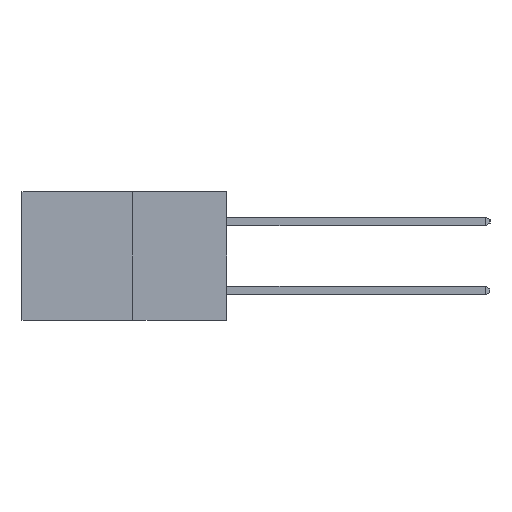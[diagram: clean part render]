
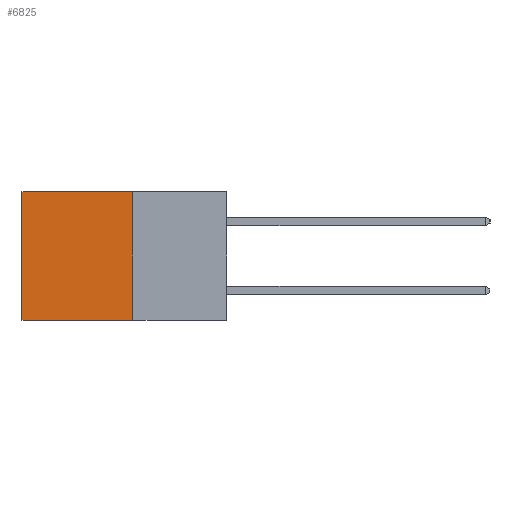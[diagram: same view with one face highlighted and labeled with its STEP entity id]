
A CAD part, left-side view. The second image highlights one B-rep face of the part: STEP entity #6825.
In plain terms, the highlighted planar face has unit normal (-1, 0, 0).
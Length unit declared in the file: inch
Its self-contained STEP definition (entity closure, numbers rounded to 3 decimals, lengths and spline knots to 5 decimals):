
#416 = DIRECTION ( 'NONE',  ( 0., 0., -1. ) ) ;
#569 = VECTOR ( 'NONE', #416, 39.37008 ) ;
#786 = ORIENTED_EDGE ( 'NONE', *, *, #5206, .T. ) ;
#916 = CARTESIAN_POINT ( 'NONE',  ( 0.277, 0.59, 0. ) ) ;
#1398 = VERTEX_POINT ( 'NONE', #5485 ) ;
#1598 = VECTOR ( 'NONE', #9127, 39.37008 ) ;
#1998 = LINE ( 'NONE', #2437, #10944 ) ;
#2204 = DIRECTION ( 'NONE',  ( 0., 1., 0. ) ) ;
#2437 = CARTESIAN_POINT ( 'NONE',  ( 0.277, 0.27, 0. ) ) ;
#2507 = DIRECTION ( 'NONE',  ( 0., 0., -1. ) ) ;
#2519 = DIRECTION ( 'NONE',  ( 1., 0., 0. ) ) ;
#2529 = PLANE ( 'NONE',  #3953 ) ;
#2538 = CARTESIAN_POINT ( 'NONE',  ( 0.277, 0.27, -0.37 ) ) ;
#2888 = ORIENTED_EDGE ( 'NONE', *, *, #8883, .T. ) ;
#3163 = CARTESIAN_POINT ( 'NONE',  ( 0.277, 0.59, -0.37 ) ) ;
#3779 = CARTESIAN_POINT ( 'NONE',  ( 0.277, 0.27, -0.37 ) ) ;
#3953 = AXIS2_PLACEMENT_3D ( 'NONE', #2538, #2519, #2507 ) ;
#4149 = ORIENTED_EDGE ( 'NONE', *, *, #7336, .F. ) ;
#4324 = LINE ( 'NONE', #5685, #1598 ) ;
#5206 = EDGE_CURVE ( 'NONE', #1398, #8632, #1998, .T. ) ;
#5485 = CARTESIAN_POINT ( 'NONE',  ( 0.277, 0.27, 0. ) ) ;
#5685 = CARTESIAN_POINT ( 'NONE',  ( 0.277, 0.59, -0.37 ) ) ;
#6700 = VERTEX_POINT ( 'NONE', #3163 ) ;
#6825 = ADVANCED_FACE ( 'NONE', ( #10793 ), #2529, .F. ) ;
#7336 = EDGE_CURVE ( 'NONE', #1398, #9811, #7734, .T. ) ;
#7734 = LINE ( 'NONE', #10943, #569 ) ;
#7762 = CARTESIAN_POINT ( 'NONE',  ( 0.277, 0.27, -0.37 ) ) ;
#8063 = ORIENTED_EDGE ( 'NONE', *, *, #10306, .F. ) ;
#8097 = LINE ( 'NONE', #7762, #10122 ) ;
#8632 = VERTEX_POINT ( 'NONE', #916 ) ;
#8643 = DIRECTION ( 'NONE',  ( 0., 1., 0. ) ) ;
#8883 = EDGE_CURVE ( 'NONE', #8632, #6700, #4324, .T. ) ;
#9127 = DIRECTION ( 'NONE',  ( 0., 0., -1. ) ) ;
#9811 = VERTEX_POINT ( 'NONE', #3779 ) ;
#10122 = VECTOR ( 'NONE', #8643, 39.37008 ) ;
#10306 = EDGE_CURVE ( 'NONE', #9811, #6700, #8097, .T. ) ;
#10793 = FACE_OUTER_BOUND ( 'NONE', #10847, .T. ) ;
#10847 = EDGE_LOOP ( 'NONE', ( #2888, #8063, #4149, #786 ) ) ;
#10943 = CARTESIAN_POINT ( 'NONE',  ( 0.277, 0.27, -0.37 ) ) ;
#10944 = VECTOR ( 'NONE', #2204, 39.37008 ) ;
